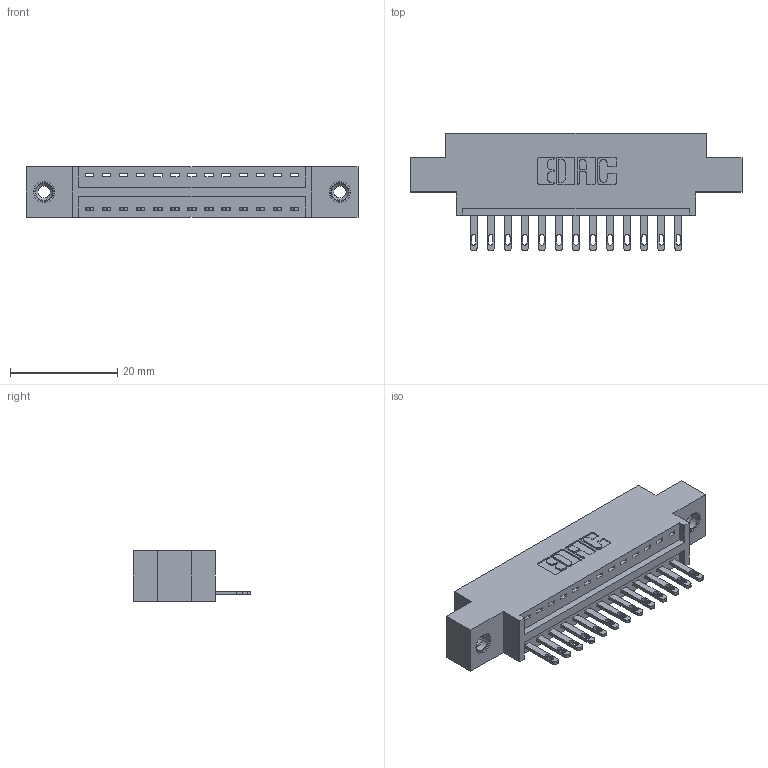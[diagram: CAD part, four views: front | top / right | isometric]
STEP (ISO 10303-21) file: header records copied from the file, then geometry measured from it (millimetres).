
FILE_DESCRIPTION (( 'STEP AP203' ), '1' );
FILE_NAME ('896-013-500-608.STEP', '2021-07-27T15:04:38', ( '' ), ( '' ), 'SwSTEP 2.0', 'SolidWorks 2020', '' );
FILE_SCHEMA (( 'CONFIG_CONTROL_DESIGN' ));
Length unit declared in the file: inch
Products named in the file (4): 345-292-001_345-293-100; 846 Part_0.170 Offset - 0.156 Dia-TI; 896-013-500-608; 345-250-001_345-250-003-102
Assembly tree (16 placements, depth 2):
  896-013-500-608
    846 Part_0.170 Offset - 0.156 Dia-TI
    345-292-001_345-293-100  x13
    345-250-001_345-250-003-102  x2
Bounding box: 61.85 x 21.84 x 9.4 mm (x, y, z)
Volume: 5567.4 mm3; surface area: 6858.1 mm2
Topology: 16 solids, 16 shells, 888 faces, 2661 edges, 1766 vertices
Faces by surface type: plane 554, cylinder 318, cone 12, torus 4
Entity records: 13220 total; most frequent: CARTESIAN_POINT 2258, ORIENTED_EDGE 2198, DIRECTION 2055, EDGE_CURVE 1099, VECTOR 891, LINE 891, VERTEX_POINT 728, AXIS2_PLACEMENT_3D 582
